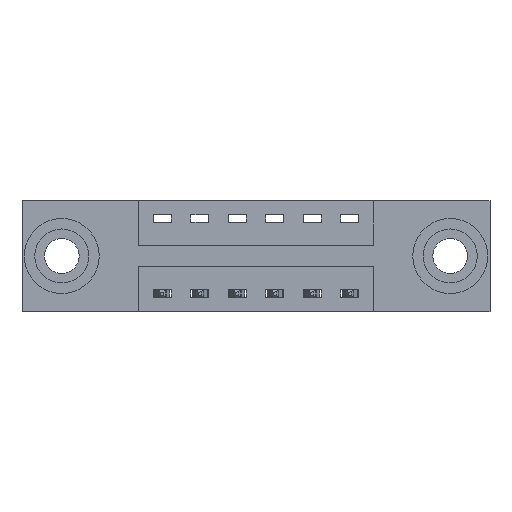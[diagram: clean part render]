
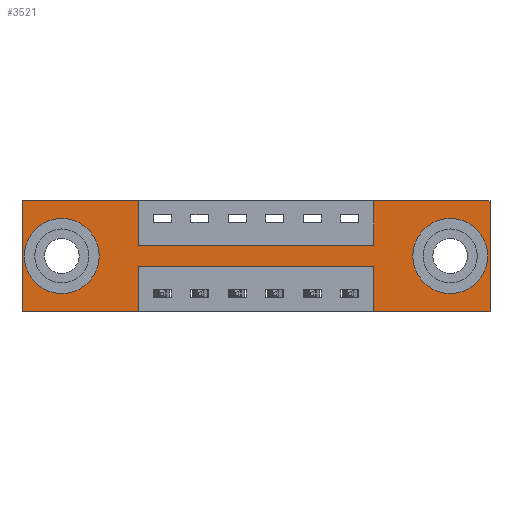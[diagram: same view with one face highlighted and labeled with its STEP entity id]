
A CAD part, front view. The second image highlights one B-rep face of the part: STEP entity #3521.
In plain terms, the highlighted planar face has unit normal (0, -1, 0).
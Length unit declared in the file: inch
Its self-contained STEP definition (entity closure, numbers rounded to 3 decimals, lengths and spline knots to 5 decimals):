
#38 = ORIENTED_EDGE ( 'NONE', *, *, #9282, .F. ) ;
#331 = CARTESIAN_POINT ( 'NONE',  ( 1.1725, 0., 0. ) ) ;
#342 = ORIENTED_EDGE ( 'NONE', *, *, #9051, .F. ) ;
#353 = AXIS2_PLACEMENT_3D ( 'NONE', #1065, #6376, #9378 ) ;
#405 = CARTESIAN_POINT ( 'NONE',  ( 1.4275, 0., -0.107 ) ) ;
#464 = ORIENTED_EDGE ( 'NONE', *, *, #5588, .F. ) ;
#498 = VERTEX_POINT ( 'NONE', #1032 ) ;
#587 = VERTEX_POINT ( 'NONE', #405 ) ;
#689 = ORIENTED_EDGE ( 'NONE', *, *, #1750, .F. ) ;
#735 = CARTESIAN_POINT ( 'NONE',  ( 0., 0., -0.37 ) ) ;
#765 = DIRECTION ( 'NONE',  ( 0., 0., -1. ) ) ;
#846 = EDGE_LOOP ( 'NONE', ( #6394, #2329 ) ) ;
#923 = EDGE_CURVE ( 'NONE', #587, #1857, #7090, .T. ) ;
#945 = EDGE_CURVE ( 'NONE', #1142, #2200, #1733, .T. ) ;
#1007 = ORIENTED_EDGE ( 'NONE', *, *, #5338, .T. ) ;
#1032 = CARTESIAN_POINT ( 'NONE',  ( 0.1325, 0., -0.107 ) ) ;
#1065 = CARTESIAN_POINT ( 'NONE',  ( 0.1325, 0., -0.185 ) ) ;
#1142 = VERTEX_POINT ( 'NONE', #2001 ) ;
#1196 = CARTESIAN_POINT ( 'NONE',  ( 1.56, 0., 0. ) ) ;
#1274 = DIRECTION ( 'NONE',  ( 0., 0., 1. ) ) ;
#1301 = DIRECTION ( 'NONE',  ( -1., 0., 0. ) ) ;
#1321 = CARTESIAN_POINT ( 'NONE',  ( 1.1725, 0., -0.37 ) ) ;
#1424 = DIRECTION ( 'NONE',  ( -1., 0., 0. ) ) ;
#1490 = VECTOR ( 'NONE', #2620, 39.37008 ) ;
#1495 = FACE_BOUND ( 'NONE', #846, .T. ) ;
#1602 = DIRECTION ( 'NONE',  ( 1., 0., 0. ) ) ;
#1733 = LINE ( 'NONE', #3074, #7097 ) ;
#1750 = EDGE_CURVE ( 'NONE', #2601, #8152, #3255, .T. ) ;
#1784 = VERTEX_POINT ( 'NONE', #3445 ) ;
#1817 = VECTOR ( 'NONE', #2142, 39.37008 ) ;
#1857 = VERTEX_POINT ( 'NONE', #8066 ) ;
#1894 = DIRECTION ( 'NONE',  ( 0., 0., 1. ) ) ;
#1918 = VERTEX_POINT ( 'NONE', #5072 ) ;
#2001 = CARTESIAN_POINT ( 'NONE',  ( 0., 0., 0. ) ) ;
#2142 = DIRECTION ( 'NONE',  ( 0., 0., -1. ) ) ;
#2147 = ORIENTED_EDGE ( 'NONE', *, *, #6598, .F. ) ;
#2200 = VERTEX_POINT ( 'NONE', #7692 ) ;
#2329 = ORIENTED_EDGE ( 'NONE', *, *, #6969, .T. ) ;
#2601 = VERTEX_POINT ( 'NONE', #9338 ) ;
#2620 = DIRECTION ( 'NONE',  ( 0., 0., -1. ) ) ;
#2713 = VERTEX_POINT ( 'NONE', #5944 ) ;
#2734 = EDGE_CURVE ( 'NONE', #4773, #1918, #8804, .T. ) ;
#2821 = PLANE ( 'NONE',  #7243 ) ;
#2832 = DIRECTION ( 'NONE',  ( 0., 0., -1. ) ) ;
#2852 = CARTESIAN_POINT ( 'NONE',  ( 1.1725, 0., -0.37 ) ) ;
#2968 = CARTESIAN_POINT ( 'NONE',  ( 1.56, 0., 0. ) ) ;
#3074 = CARTESIAN_POINT ( 'NONE',  ( 0., 0., 0. ) ) ;
#3255 = LINE ( 'NONE', #331, #5582 ) ;
#3256 = DIRECTION ( 'NONE',  ( 1., 0., 0. ) ) ;
#3445 = CARTESIAN_POINT ( 'NONE',  ( 0.3875, 0., -0.22 ) ) ;
#3492 = VECTOR ( 'NONE', #3256, 39.37008 ) ;
#3521 = ADVANCED_FACE ( 'NONE', ( #1495, #8784, #5870 ), #2821, .T. ) ;
#3522 = VERTEX_POINT ( 'NONE', #9519 ) ;
#3577 = VECTOR ( 'NONE', #1424, 39.37008 ) ;
#3617 = CIRCLE ( 'NONE', #353, 0.078 ) ;
#3668 = EDGE_CURVE ( 'NONE', #1784, #4773, #4554, .T. ) ;
#3715 = EDGE_CURVE ( 'NONE', #3522, #498, #8356, .T. ) ;
#3818 = DIRECTION ( 'NONE',  ( 0., 0., -1. ) ) ;
#3970 = VERTEX_POINT ( 'NONE', #2852 ) ;
#3976 = LINE ( 'NONE', #7565, #3492 ) ;
#4077 = EDGE_LOOP ( 'NONE', ( #1007, #8172 ) ) ;
#4126 = CARTESIAN_POINT ( 'NONE',  ( 1.1725, 0., 0. ) ) ;
#4213 = VERTEX_POINT ( 'NONE', #6797 ) ;
#4381 = DIRECTION ( 'NONE',  ( 0., 1., 0. ) ) ;
#4392 = LINE ( 'NONE', #1321, #6984 ) ;
#4523 = ORIENTED_EDGE ( 'NONE', *, *, #7263, .F. ) ;
#4554 = LINE ( 'NONE', #8444, #7092 ) ;
#4580 = VECTOR ( 'NONE', #1894, 39.37008 ) ;
#4652 = DIRECTION ( 'NONE',  ( 0., 1., 0. ) ) ;
#4674 = EDGE_CURVE ( 'NONE', #1918, #1142, #6464, .T. ) ;
#4710 = DIRECTION ( 'NONE',  ( 0., 0., -1. ) ) ;
#4773 = VERTEX_POINT ( 'NONE', #5735 ) ;
#4835 = VERTEX_POINT ( 'NONE', #5257 ) ;
#5018 = DIRECTION ( 'NONE',  ( 0., -1., 0. ) ) ;
#5072 = CARTESIAN_POINT ( 'NONE',  ( 0., 0., -0.37 ) ) ;
#5079 = CIRCLE ( 'NONE', #9286, 0.078 ) ;
#5094 = VECTOR ( 'NONE', #7343, 39.37008 ) ;
#5257 = CARTESIAN_POINT ( 'NONE',  ( 1.1725, 0., -0.22 ) ) ;
#5338 = EDGE_CURVE ( 'NONE', #498, #3522, #3617, .T. ) ;
#5582 = VECTOR ( 'NONE', #6425, 39.37008 ) ;
#5588 = EDGE_CURVE ( 'NONE', #4213, #3970, #5778, .T. ) ;
#5704 = DIRECTION ( 'NONE',  ( -1., 0., 0. ) ) ;
#5735 = CARTESIAN_POINT ( 'NONE',  ( 0.3875, 0., -0.37 ) ) ;
#5778 = LINE ( 'NONE', #8016, #8350 ) ;
#5809 = AXIS2_PLACEMENT_3D ( 'NONE', #6807, #4652, #7638 ) ;
#5870 = FACE_OUTER_BOUND ( 'NONE', #7486, .T. ) ;
#5944 = CARTESIAN_POINT ( 'NONE',  ( 0.3875, 0., -0.15 ) ) ;
#6014 = LINE ( 'NONE', #2968, #1817 ) ;
#6311 = CARTESIAN_POINT ( 'NONE',  ( 0.3875, 0., 0. ) ) ;
#6376 = DIRECTION ( 'NONE',  ( 0., 1., 0. ) ) ;
#6394 = ORIENTED_EDGE ( 'NONE', *, *, #923, .T. ) ;
#6425 = DIRECTION ( 'NONE',  ( 0., 0., 1. ) ) ;
#6443 = LINE ( 'NONE', #8581, #6975 ) ;
#6464 = LINE ( 'NONE', #9317, #4580 ) ;
#6521 = CARTESIAN_POINT ( 'NONE',  ( 0., 0., -0.37 ) ) ;
#6598 = EDGE_CURVE ( 'NONE', #2713, #2601, #3976, .T. ) ;
#6797 = CARTESIAN_POINT ( 'NONE',  ( 1.56, 0., -0.37 ) ) ;
#6807 = CARTESIAN_POINT ( 'NONE',  ( 0.1325, 0., -0.185 ) ) ;
#6969 = EDGE_CURVE ( 'NONE', #1857, #587, #5079, .T. ) ;
#6975 = VECTOR ( 'NONE', #5704, 39.37008 ) ;
#6984 = VECTOR ( 'NONE', #1274, 39.37008 ) ;
#7090 = CIRCLE ( 'NONE', #9583, 0.078 ) ;
#7092 = VECTOR ( 'NONE', #3818, 39.37008 ) ;
#7097 = VECTOR ( 'NONE', #1602, 39.37008 ) ;
#7214 = ORIENTED_EDGE ( 'NONE', *, *, #2734, .F. ) ;
#7243 = AXIS2_PLACEMENT_3D ( 'NONE', #6521, #5018, #765 ) ;
#7263 = EDGE_CURVE ( 'NONE', #2200, #2713, #7963, .T. ) ;
#7343 = DIRECTION ( 'NONE',  ( 1., 0., 0. ) ) ;
#7472 = ORIENTED_EDGE ( 'NONE', *, *, #945, .F. ) ;
#7486 = EDGE_LOOP ( 'NONE', ( #8017, #342, #38, #464, #7596, #7873, #689, #2147, #4523, #7472, #7980, #7214 ) ) ;
#7492 = CARTESIAN_POINT ( 'NONE',  ( 0., 0., 0. ) ) ;
#7565 = CARTESIAN_POINT ( 'NONE',  ( 0.3875, 0., -0.15 ) ) ;
#7596 = ORIENTED_EDGE ( 'NONE', *, *, #8306, .F. ) ;
#7638 = DIRECTION ( 'NONE',  ( 0., 0., 1. ) ) ;
#7692 = CARTESIAN_POINT ( 'NONE',  ( 0.3875, 0., 0. ) ) ;
#7746 = CARTESIAN_POINT ( 'NONE',  ( 1.4275, 0., -0.185 ) ) ;
#7873 = ORIENTED_EDGE ( 'NONE', *, *, #8677, .F. ) ;
#7963 = LINE ( 'NONE', #6311, #1490 ) ;
#7980 = ORIENTED_EDGE ( 'NONE', *, *, #4674, .F. ) ;
#8016 = CARTESIAN_POINT ( 'NONE',  ( 0., 0., -0.37 ) ) ;
#8017 = ORIENTED_EDGE ( 'NONE', *, *, #3668, .F. ) ;
#8066 = CARTESIAN_POINT ( 'NONE',  ( 1.4275, 0., -0.263 ) ) ;
#8152 = VERTEX_POINT ( 'NONE', #4126 ) ;
#8172 = ORIENTED_EDGE ( 'NONE', *, *, #3715, .T. ) ;
#8306 = EDGE_CURVE ( 'NONE', #8602, #4213, #6014, .T. ) ;
#8350 = VECTOR ( 'NONE', #1301, 39.37008 ) ;
#8356 = CIRCLE ( 'NONE', #5809, 0.078 ) ;
#8444 = CARTESIAN_POINT ( 'NONE',  ( 0.3875, 0., -0.37 ) ) ;
#8581 = CARTESIAN_POINT ( 'NONE',  ( 0.3875, 0., -0.22 ) ) ;
#8602 = VERTEX_POINT ( 'NONE', #1196 ) ;
#8677 = EDGE_CURVE ( 'NONE', #8152, #8602, #9549, .T. ) ;
#8784 = FACE_BOUND ( 'NONE', #4077, .T. ) ;
#8804 = LINE ( 'NONE', #735, #3577 ) ;
#8940 = CARTESIAN_POINT ( 'NONE',  ( 1.4275, 0., -0.185 ) ) ;
#9051 = EDGE_CURVE ( 'NONE', #4835, #1784, #6443, .T. ) ;
#9122 = DIRECTION ( 'NONE',  ( 0., 1., 0. ) ) ;
#9282 = EDGE_CURVE ( 'NONE', #3970, #4835, #4392, .T. ) ;
#9286 = AXIS2_PLACEMENT_3D ( 'NONE', #7746, #9122, #4710 ) ;
#9317 = CARTESIAN_POINT ( 'NONE',  ( 0., 0., 0. ) ) ;
#9338 = CARTESIAN_POINT ( 'NONE',  ( 1.1725, 0., -0.15 ) ) ;
#9378 = DIRECTION ( 'NONE',  ( 0., 0., 1. ) ) ;
#9519 = CARTESIAN_POINT ( 'NONE',  ( 0.1325, 0., -0.263 ) ) ;
#9549 = LINE ( 'NONE', #7492, #5094 ) ;
#9583 = AXIS2_PLACEMENT_3D ( 'NONE', #8940, #4381, #2832 ) ;
